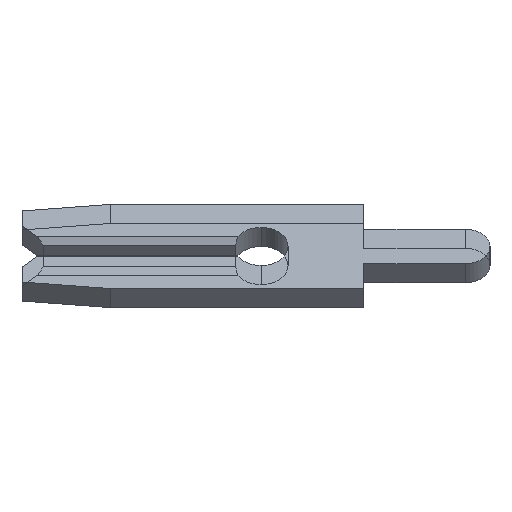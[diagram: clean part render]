
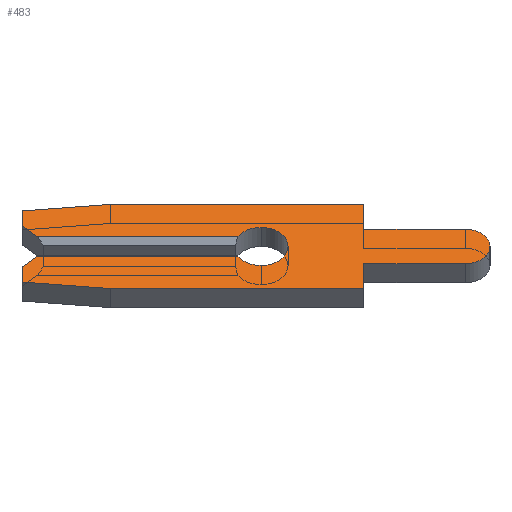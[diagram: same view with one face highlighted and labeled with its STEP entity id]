
A CAD part, left-side view. The second image highlights one B-rep face of the part: STEP entity #483.
In plain terms, the highlighted face is planar.
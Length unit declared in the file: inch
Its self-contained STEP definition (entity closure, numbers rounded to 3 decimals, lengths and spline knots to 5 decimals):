
#9 = VERTEX_POINT ( 'NONE', #2064 ) ;
#29 = DIRECTION ( 'NONE',  ( -1., 0., 0. ) ) ;
#69 = VERTEX_POINT ( 'NONE', #2437 ) ;
#83 = CARTESIAN_POINT ( 'NONE',  ( -0.013, -0.099, -0.0575 ) ) ;
#122 = VECTOR ( 'NONE', #703, 39.37008 ) ;
#123 = EDGE_CURVE ( 'NONE', #2526, #2048, #2404, .T. ) ;
#148 = CARTESIAN_POINT ( 'NONE',  ( -0.013, 0.231, 0.04857 ) ) ;
#188 = ORIENTED_EDGE ( 'NONE', *, *, #577, .F. ) ;
#215 = LINE ( 'NONE', #1555, #575 ) ;
#256 = VECTOR ( 'NONE', #774, 39.37008 ) ;
#257 = CARTESIAN_POINT ( 'NONE',  ( -0.013, -0.099, 0.0235 ) ) ;
#290 = VERTEX_POINT ( 'NONE', #257 ) ;
#292 = DIRECTION ( 'NONE',  ( 0., 0., -1. ) ) ;
#324 = DIRECTION ( 'NONE',  ( 0., -0.707, 0.707 ) ) ;
#340 = CARTESIAN_POINT ( 'NONE',  ( -0.013, 0.146, -0.0575 ) ) ;
#359 = DIRECTION ( 'NONE',  ( 0., 1., 0. ) ) ;
#401 = EDGE_CURVE ( 'NONE', #1070, #2048, #2524, .T. ) ;
#419 = LINE ( 'NONE', #1764, #122 ) ;
#421 = ORIENTED_EDGE ( 'NONE', *, *, #771, .F. ) ;
#440 = EDGE_CURVE ( 'NONE', #833, #998, #1198, .T. ) ;
#443 = VERTEX_POINT ( 'NONE', #1172 ) ;
#450 = VECTOR ( 'NONE', #1637, 39.37008 ) ;
#456 = DIRECTION ( 'NONE',  ( -1., 0., 0. ) ) ;
#477 = CARTESIAN_POINT ( 'NONE',  ( -0.013, 0.231, 0.028 ) ) ;
#483 = ADVANCED_FACE ( 'NONE', ( #1959 ), #2344, .F. ) ;
#485 = DIRECTION ( 'NONE',  ( 0., -1., 0. ) ) ;
#513 = ORIENTED_EDGE ( 'NONE', *, *, #2562, .F. ) ;
#518 = ORIENTED_EDGE ( 'NONE', *, *, #682, .F. ) ;
#575 = VECTOR ( 'NONE', #485, 39.37008 ) ;
#577 = EDGE_CURVE ( 'NONE', #1361, #878, #2239, .T. ) ;
#584 = LINE ( 'NONE', #754, #947 ) ;
#611 = LINE ( 'NONE', #972, #2560 ) ;
#618 = CARTESIAN_POINT ( 'NONE',  ( -0.013, 0.2105, 0.0075 ) ) ;
#628 = CARTESIAN_POINT ( 'NONE',  ( -0.013, 0.231, -0.04857 ) ) ;
#629 = EDGE_CURVE ( 'NONE', #69, #1861, #1420, .T. ) ;
#645 = EDGE_LOOP ( 'NONE', ( #1613, #1025, #2241, #1734, #1851, #513, #518, #2151, #1221, #188, #1590, #2021, #421, #838, #2561, #1480, #2380, #801 ) ) ;
#651 = DIRECTION ( 'NONE',  ( 0., 0., -1. ) ) ;
#667 = DIRECTION ( 'NONE',  ( 0., 0., -1. ) ) ;
#677 = CARTESIAN_POINT ( 'NONE',  ( -0.013, 0., 0. ) ) ;
#682 = EDGE_CURVE ( 'NONE', #1549, #443, #419, .T. ) ;
#703 = DIRECTION ( 'NONE',  ( 0., 0., 1. ) ) ;
#705 = VECTOR ( 'NONE', #2557, 39.37008 ) ;
#741 = VECTOR ( 'NONE', #1286, 39.37008 ) ;
#754 = CARTESIAN_POINT ( 'NONE',  ( -0.013, 0.2105, -0.0075 ) ) ;
#764 = DIRECTION ( 'NONE',  ( 1., 0., 0. ) ) ;
#771 = EDGE_CURVE ( 'NONE', #290, #2273, #611, .T. ) ;
#773 = VECTOR ( 'NONE', #1939, 39.37008 ) ;
#774 = DIRECTION ( 'NONE',  ( 0., 0., 1. ) ) ;
#801 = ORIENTED_EDGE ( 'NONE', *, *, #1375, .F. ) ;
#805 = VECTOR ( 'NONE', #1687, 39.37008 ) ;
#833 = VERTEX_POINT ( 'NONE', #477 ) ;
#838 = ORIENTED_EDGE ( 'NONE', *, *, #2101, .F. ) ;
#878 = VERTEX_POINT ( 'NONE', #1006 ) ;
#930 = EDGE_CURVE ( 'NONE', #1251, #1798, #1669, .T. ) ;
#943 = LINE ( 'NONE', #148, #741 ) ;
#947 = VECTOR ( 'NONE', #324, 39.37008 ) ;
#971 = CIRCLE ( 'NONE', #1835, 0.026 ) ;
#972 = CARTESIAN_POINT ( 'NONE',  ( -0.013, -0.099, 0.0235 ) ) ;
#998 = VERTEX_POINT ( 'NONE', #2602 ) ;
#1006 = CARTESIAN_POINT ( 'NONE',  ( -0.013, -0.099, -0.0575 ) ) ;
#1025 = ORIENTED_EDGE ( 'NONE', *, *, #123, .F. ) ;
#1070 = VERTEX_POINT ( 'NONE', #1940 ) ;
#1115 = EDGE_CURVE ( 'NONE', #998, #69, #943, .T. ) ;
#1128 = VECTOR ( 'NONE', #2278, 39.37008 ) ;
#1166 = DIRECTION ( 'NONE',  ( 0., 0., 1. ) ) ;
#1172 = CARTESIAN_POINT ( 'NONE',  ( -0.013, 0.231, -0.028 ) ) ;
#1198 = LINE ( 'NONE', #2181, #256 ) ;
#1221 = ORIENTED_EDGE ( 'NONE', *, *, #1233, .F. ) ;
#1233 = EDGE_CURVE ( 'NONE', #878, #2407, #1526, .T. ) ;
#1251 = VERTEX_POINT ( 'NONE', #1827 ) ;
#1253 = LINE ( 'NONE', #1515, #705 ) ;
#1286 = DIRECTION ( 'NONE',  ( 0., -0.995, 0.105 ) ) ;
#1343 = CARTESIAN_POINT ( 'NONE',  ( -0.013, 0.02252, 0.013 ) ) ;
#1359 = AXIS2_PLACEMENT_3D ( 'NONE', #2225, #1394, #1620 ) ;
#1361 = VERTEX_POINT ( 'NONE', #1662 ) ;
#1364 = CARTESIAN_POINT ( 'NONE',  ( -0.013, 0., 0. ) ) ;
#1375 = EDGE_CURVE ( 'NONE', #1070, #833, #1586, .T. ) ;
#1391 = CARTESIAN_POINT ( 'NONE',  ( -0.013, -0.1975, 0. ) ) ;
#1394 = DIRECTION ( 'NONE',  ( -1., 0., 0. ) ) ;
#1420 = LINE ( 'NONE', #1924, #2595 ) ;
#1480 = ORIENTED_EDGE ( 'NONE', *, *, #1115, .F. ) ;
#1515 = CARTESIAN_POINT ( 'NONE',  ( -0.013, -0.099, -0.0235 ) ) ;
#1526 = LINE ( 'NONE', #340, #2495 ) ;
#1527 = DIRECTION ( 'NONE',  ( 0., -1., 0. ) ) ;
#1549 = VERTEX_POINT ( 'NONE', #628 ) ;
#1555 = CARTESIAN_POINT ( 'NONE',  ( -0.013, 0., -0.013 ) ) ;
#1586 = LINE ( 'NONE', #618, #450 ) ;
#1590 = ORIENTED_EDGE ( 'NONE', *, *, #2236, .F. ) ;
#1613 = ORIENTED_EDGE ( 'NONE', *, *, #401, .T. ) ;
#1620 = DIRECTION ( 'NONE',  ( 0., 0., -1. ) ) ;
#1637 = DIRECTION ( 'NONE',  ( 0., 0.707, 0.707 ) ) ;
#1662 = CARTESIAN_POINT ( 'NONE',  ( -0.013, -0.099, -0.0235 ) ) ;
#1668 = LINE ( 'NONE', #2086, #1128 ) ;
#1669 = CIRCLE ( 'NONE', #1359, 0.026 ) ;
#1687 = DIRECTION ( 'NONE',  ( 0., -1., 0. ) ) ;
#1703 = VECTOR ( 'NONE', #292, 39.37008 ) ;
#1710 = DIRECTION ( 'NONE',  ( 0., 0., -1. ) ) ;
#1729 = EDGE_CURVE ( 'NONE', #1798, #2526, #971, .T. ) ;
#1734 = ORIENTED_EDGE ( 'NONE', *, *, #930, .F. ) ;
#1764 = CARTESIAN_POINT ( 'NONE',  ( -0.013, 0.231, -0.028 ) ) ;
#1798 = VERTEX_POINT ( 'NONE', #2289 ) ;
#1827 = CARTESIAN_POINT ( 'NONE',  ( -0.013, 0.02252, -0.013 ) ) ;
#1835 = AXIS2_PLACEMENT_3D ( 'NONE', #2480, #29, #651 ) ;
#1851 = ORIENTED_EDGE ( 'NONE', *, *, #1955, .F. ) ;
#1861 = VERTEX_POINT ( 'NONE', #2080 ) ;
#1865 = EDGE_CURVE ( 'NONE', #2407, #1549, #1668, .T. ) ;
#1924 = CARTESIAN_POINT ( 'NONE',  ( -0.013, 0.146, 0.0575 ) ) ;
#1934 = CARTESIAN_POINT ( 'NONE',  ( -0.013, 0., 0.026 ) ) ;
#1939 = DIRECTION ( 'NONE',  ( 0., 0., -1. ) ) ;
#1940 = CARTESIAN_POINT ( 'NONE',  ( -0.013, 0.216, 0.013 ) ) ;
#1955 = EDGE_CURVE ( 'NONE', #2275, #1251, #215, .T. ) ;
#1959 = FACE_OUTER_BOUND ( 'NONE', #645, .T. ) ;
#1971 = DIRECTION ( 'NONE',  ( 0., -1., 0. ) ) ;
#2021 = ORIENTED_EDGE ( 'NONE', *, *, #2504, .F. ) ;
#2048 = VERTEX_POINT ( 'NONE', #1343 ) ;
#2064 = CARTESIAN_POINT ( 'NONE',  ( -0.013, -0.1975, -0.0235 ) ) ;
#2080 = CARTESIAN_POINT ( 'NONE',  ( -0.013, -0.099, 0.0575 ) ) ;
#2086 = CARTESIAN_POINT ( 'NONE',  ( -0.013, 0.231, -0.04857 ) ) ;
#2101 = EDGE_CURVE ( 'NONE', #1861, #290, #2402, .T. ) ;
#2134 = DIRECTION ( 'NONE',  ( 1., 0., 0. ) ) ;
#2141 = CARTESIAN_POINT ( 'NONE',  ( -0.013, -0.1975, 0.0235 ) ) ;
#2146 = CIRCLE ( 'NONE', #2395, 0.0235 ) ;
#2151 = ORIENTED_EDGE ( 'NONE', *, *, #1865, .F. ) ;
#2181 = CARTESIAN_POINT ( 'NONE',  ( -0.013, 0.231, 0.028 ) ) ;
#2225 = CARTESIAN_POINT ( 'NONE',  ( -0.013, 0., 0. ) ) ;
#2236 = EDGE_CURVE ( 'NONE', #9, #1361, #1253, .T. ) ;
#2239 = LINE ( 'NONE', #83, #1703 ) ;
#2241 = ORIENTED_EDGE ( 'NONE', *, *, #1729, .F. ) ;
#2273 = VERTEX_POINT ( 'NONE', #2141 ) ;
#2275 = VERTEX_POINT ( 'NONE', #2357 ) ;
#2278 = DIRECTION ( 'NONE',  ( 0., 0.995, 0.105 ) ) ;
#2281 = CARTESIAN_POINT ( 'NONE',  ( -0.013, 0.231, 0.013 ) ) ;
#2289 = CARTESIAN_POINT ( 'NONE',  ( -0.013, 0., -0.026 ) ) ;
#2342 = CARTESIAN_POINT ( 'NONE',  ( -0.013, 0.146, -0.0575 ) ) ;
#2344 = PLANE ( 'NONE',  #2543 ) ;
#2357 = CARTESIAN_POINT ( 'NONE',  ( -0.013, 0.216, -0.013 ) ) ;
#2380 = ORIENTED_EDGE ( 'NONE', *, *, #440, .F. ) ;
#2395 = AXIS2_PLACEMENT_3D ( 'NONE', #1391, #764, #1166 ) ;
#2402 = LINE ( 'NONE', #2545, #773 ) ;
#2404 = CIRCLE ( 'NONE', #2411, 0.026 ) ;
#2407 = VERTEX_POINT ( 'NONE', #2342 ) ;
#2411 = AXIS2_PLACEMENT_3D ( 'NONE', #677, #456, #667 ) ;
#2437 = CARTESIAN_POINT ( 'NONE',  ( -0.013, 0.146, 0.0575 ) ) ;
#2480 = CARTESIAN_POINT ( 'NONE',  ( -0.013, 0., 0. ) ) ;
#2495 = VECTOR ( 'NONE', #359, 39.37008 ) ;
#2504 = EDGE_CURVE ( 'NONE', #2273, #9, #2146, .T. ) ;
#2524 = LINE ( 'NONE', #2281, #805 ) ;
#2526 = VERTEX_POINT ( 'NONE', #1934 ) ;
#2543 = AXIS2_PLACEMENT_3D ( 'NONE', #1364, #2134, #1710 ) ;
#2545 = CARTESIAN_POINT ( 'NONE',  ( -0.013, -0.099, 0.0575 ) ) ;
#2557 = DIRECTION ( 'NONE',  ( 0., 1., 0. ) ) ;
#2560 = VECTOR ( 'NONE', #1971, 39.37008 ) ;
#2561 = ORIENTED_EDGE ( 'NONE', *, *, #629, .F. ) ;
#2562 = EDGE_CURVE ( 'NONE', #443, #2275, #584, .T. ) ;
#2595 = VECTOR ( 'NONE', #1527, 39.37008 ) ;
#2602 = CARTESIAN_POINT ( 'NONE',  ( -0.013, 0.231, 0.04857 ) ) ;
